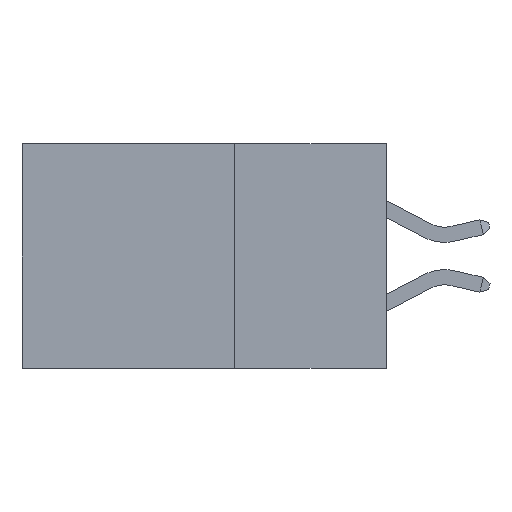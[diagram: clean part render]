
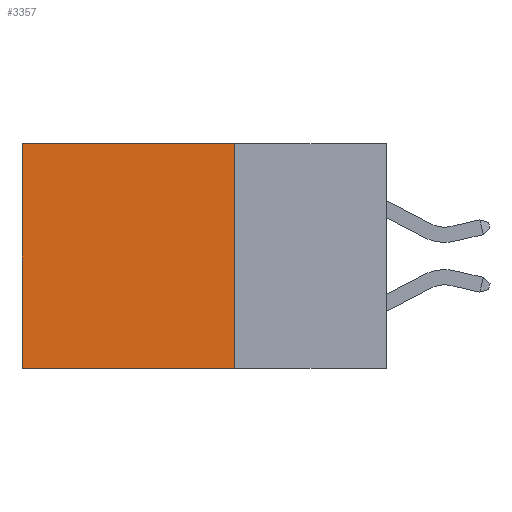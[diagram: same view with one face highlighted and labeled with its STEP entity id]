
A CAD part, left-side view. The second image highlights one B-rep face of the part: STEP entity #3357.
In plain terms, the highlighted planar face has unit normal (-1, 0, 0).
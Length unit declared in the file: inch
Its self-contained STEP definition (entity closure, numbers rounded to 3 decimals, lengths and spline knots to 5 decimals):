
#10 = AXIS2_PLACEMENT_3D ( 'NONE', #4240, #7069, #1157 ) ;
#1157 = DIRECTION ( 'NONE',  ( 0., 0., -1. ) ) ;
#1224 = EDGE_CURVE ( 'NONE', #9518, #7123, #1363, .T. ) ;
#1293 = DIRECTION ( 'NONE',  ( 0., 0., -1. ) ) ;
#1363 = LINE ( 'NONE', #7631, #9127 ) ;
#1854 = EDGE_CURVE ( 'NONE', #7123, #8764, #5251, .T. ) ;
#1910 = DIRECTION ( 'NONE',  ( 0., 1., 0. ) ) ;
#2730 = ORIENTED_EDGE ( 'NONE', *, *, #7565, .F. ) ;
#3197 = PLANE ( 'NONE',  #10 ) ;
#3357 = ADVANCED_FACE ( 'NONE', ( #5958 ), #3197, .F. ) ;
#4024 = CARTESIAN_POINT ( 'NONE',  ( 0.2615, 0.6, -0.37 ) ) ;
#4240 = CARTESIAN_POINT ( 'NONE',  ( 0.2615, 0.25, -0.37 ) ) ;
#4287 = EDGE_CURVE ( 'NONE', #9518, #7835, #9666, .T. ) ;
#5161 = CARTESIAN_POINT ( 'NONE',  ( 0.2615, 0.25, 0. ) ) ;
#5251 = LINE ( 'NONE', #10155, #7481 ) ;
#5275 = ORIENTED_EDGE ( 'NONE', *, *, #1224, .T. ) ;
#5708 = ORIENTED_EDGE ( 'NONE', *, *, #4287, .F. ) ;
#5958 = FACE_OUTER_BOUND ( 'NONE', #10144, .T. ) ;
#6499 = ORIENTED_EDGE ( 'NONE', *, *, #1854, .T. ) ;
#7069 = DIRECTION ( 'NONE',  ( 1., 0., 0. ) ) ;
#7109 = CARTESIAN_POINT ( 'NONE',  ( 0.2615, 0.25, -0.37 ) ) ;
#7123 = VERTEX_POINT ( 'NONE', #9779 ) ;
#7136 = VECTOR ( 'NONE', #1293, 39.37008 ) ;
#7481 = VECTOR ( 'NONE', #10398, 39.37008 ) ;
#7565 = EDGE_CURVE ( 'NONE', #7835, #8764, #11583, .T. ) ;
#7631 = CARTESIAN_POINT ( 'NONE',  ( 0.2615, 0.25, 0. ) ) ;
#7672 = DIRECTION ( 'NONE',  ( 0., 1., 0. ) ) ;
#7835 = VERTEX_POINT ( 'NONE', #7109 ) ;
#8635 = CARTESIAN_POINT ( 'NONE',  ( 0.2615, 0.25, -0.37 ) ) ;
#8764 = VERTEX_POINT ( 'NONE', #4024 ) ;
#9127 = VECTOR ( 'NONE', #7672, 39.37008 ) ;
#9187 = VECTOR ( 'NONE', #1910, 39.37008 ) ;
#9518 = VERTEX_POINT ( 'NONE', #5161 ) ;
#9666 = LINE ( 'NONE', #10900, #7136 ) ;
#9779 = CARTESIAN_POINT ( 'NONE',  ( 0.2615, 0.6, 0. ) ) ;
#10144 = EDGE_LOOP ( 'NONE', ( #6499, #2730, #5708, #5275 ) ) ;
#10155 = CARTESIAN_POINT ( 'NONE',  ( 0.2615, 0.6, -0.37 ) ) ;
#10398 = DIRECTION ( 'NONE',  ( 0., 0., -1. ) ) ;
#10900 = CARTESIAN_POINT ( 'NONE',  ( 0.2615, 0.25, -0.37 ) ) ;
#11583 = LINE ( 'NONE', #8635, #9187 ) ;
